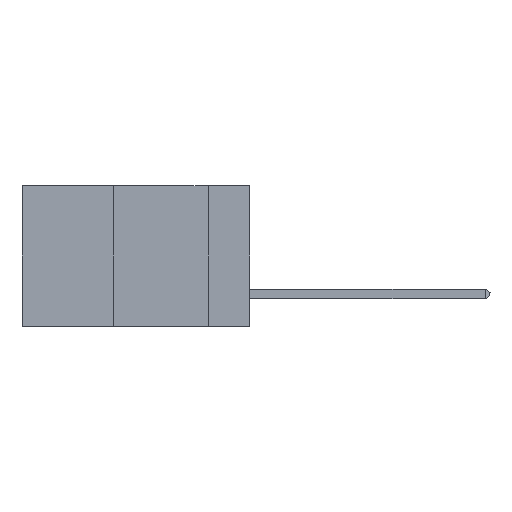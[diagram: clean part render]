
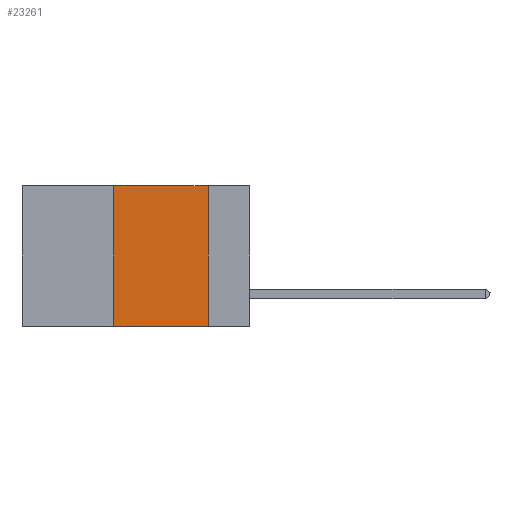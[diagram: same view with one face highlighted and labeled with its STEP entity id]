
A CAD part, left-side view. The second image highlights one B-rep face of the part: STEP entity #23261.
In plain terms, the highlighted planar face has unit normal (-1, 0, 0).
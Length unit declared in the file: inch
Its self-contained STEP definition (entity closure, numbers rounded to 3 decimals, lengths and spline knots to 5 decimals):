
#561 = VERTEX_POINT ( 'NONE', #12503 ) ;
#1251 = CARTESIAN_POINT ( 'NONE',  ( 0., 0.6, -0.37 ) ) ;
#2482 = ORIENTED_EDGE ( 'NONE', *, *, #11748, .T. ) ;
#3801 = VERTEX_POINT ( 'NONE', #11398 ) ;
#4904 = CARTESIAN_POINT ( 'NONE',  ( 0., 0.11, 0. ) ) ;
#5052 = CARTESIAN_POINT ( 'NONE',  ( 0., 0.11, 0. ) ) ;
#5573 = LINE ( 'NONE', #5052, #23878 ) ;
#8125 = VECTOR ( 'NONE', #19018, 39.37008 ) ;
#9112 = EDGE_CURVE ( 'NONE', #22792, #561, #24992, .T. ) ;
#9522 = DIRECTION ( 'NONE',  ( 0., 0., -1. ) ) ;
#9849 = DIRECTION ( 'NONE',  ( 0., 0., -1. ) ) ;
#10460 = CARTESIAN_POINT ( 'NONE',  ( 0., 0.6, 0. ) ) ;
#10563 = DIRECTION ( 'NONE',  ( 0., -1., 0. ) ) ;
#10747 = ORIENTED_EDGE ( 'NONE', *, *, #11150, .F. ) ;
#11150 = EDGE_CURVE ( 'NONE', #561, #14450, #11569, .T. ) ;
#11398 = CARTESIAN_POINT ( 'NONE',  ( 0., 0.11, -0.37 ) ) ;
#11542 = VECTOR ( 'NONE', #24362, 39.37008 ) ;
#11569 = LINE ( 'NONE', #10460, #16833 ) ;
#11748 = EDGE_CURVE ( 'NONE', #22792, #3801, #23432, .T. ) ;
#12340 = EDGE_LOOP ( 'NONE', ( #23330, #10747, #19498, #2482 ) ) ;
#12503 = CARTESIAN_POINT ( 'NONE',  ( 0., 0.36, 0. ) ) ;
#14450 = VERTEX_POINT ( 'NONE', #4904 ) ;
#15233 = FACE_OUTER_BOUND ( 'NONE', #12340, .T. ) ;
#16833 = VECTOR ( 'NONE', #10563, 39.37008 ) ;
#19018 = DIRECTION ( 'NONE',  ( 0., 0., 1. ) ) ;
#19498 = ORIENTED_EDGE ( 'NONE', *, *, #9112, .F. ) ;
#20450 = CARTESIAN_POINT ( 'NONE',  ( 0., 0.6, 0. ) ) ;
#22792 = VERTEX_POINT ( 'NONE', #26057 ) ;
#22943 = DIRECTION ( 'NONE',  ( 1., 0., 0. ) ) ;
#23261 = ADVANCED_FACE ( 'NONE', ( #15233 ), #28951, .F. ) ;
#23330 = ORIENTED_EDGE ( 'NONE', *, *, #24375, .F. ) ;
#23432 = LINE ( 'NONE', #1251, #11542 ) ;
#23878 = VECTOR ( 'NONE', #9849, 39.37008 ) ;
#24362 = DIRECTION ( 'NONE',  ( 0., -1., 0. ) ) ;
#24375 = EDGE_CURVE ( 'NONE', #14450, #3801, #5573, .T. ) ;
#24992 = LINE ( 'NONE', #26095, #8125 ) ;
#26057 = CARTESIAN_POINT ( 'NONE',  ( 0., 0.36, -0.37 ) ) ;
#26095 = CARTESIAN_POINT ( 'NONE',  ( 0., 0.36, 0. ) ) ;
#27153 = AXIS2_PLACEMENT_3D ( 'NONE', #20450, #22943, #9522 ) ;
#28951 = PLANE ( 'NONE',  #27153 ) ;
